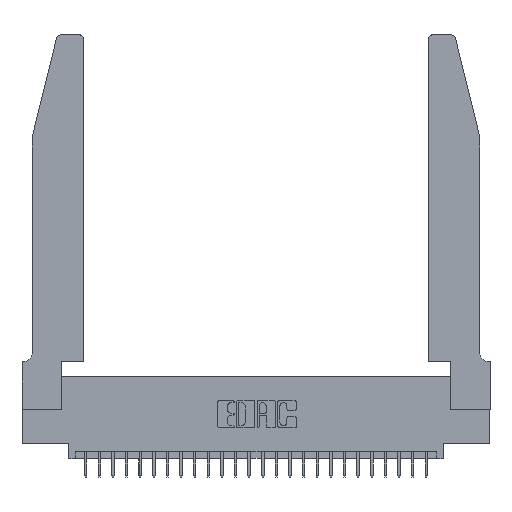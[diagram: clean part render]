
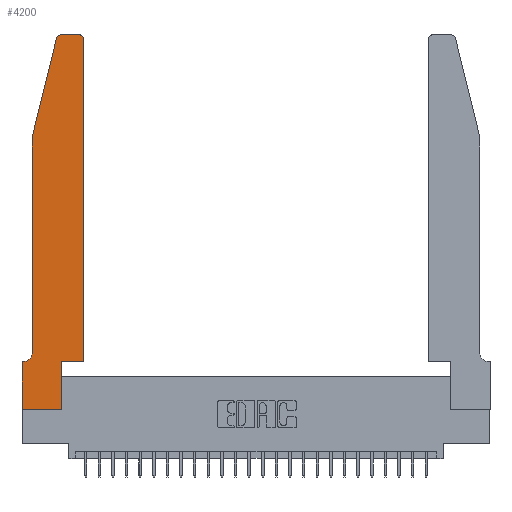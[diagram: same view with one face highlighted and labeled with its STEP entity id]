
A CAD part, top view. The second image highlights one B-rep face of the part: STEP entity #4200.
In plain terms, the highlighted planar face has unit normal (0, 0, 1).
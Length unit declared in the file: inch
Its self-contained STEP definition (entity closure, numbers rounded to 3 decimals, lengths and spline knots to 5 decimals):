
#286 = CARTESIAN_POINT ( 'NONE',  ( 0.4505, 0.35, 0.37 ) ) ;
#693 = ORIENTED_EDGE ( 'NONE', *, *, #15158, .T. ) ;
#902 = EDGE_CURVE ( 'NONE', #25947, #24993, #27378, .T. ) ;
#947 = CARTESIAN_POINT ( 'NONE',  ( 0.0755, 0.42, 0.37 ) ) ;
#1676 = VECTOR ( 'NONE', #17549, 39.37008 ) ;
#1824 = EDGE_CURVE ( 'NONE', #17527, #2844, #10276, .T. ) ;
#1993 = CARTESIAN_POINT ( 'NONE',  ( 0., 0., 0.37 ) ) ;
#2123 = ORIENTED_EDGE ( 'NONE', *, *, #1824, .T. ) ;
#2176 = DIRECTION ( 'NONE',  ( 0., -1., 0. ) ) ;
#2195 = VERTEX_POINT ( 'NONE', #15216 ) ;
#2312 = ORIENTED_EDGE ( 'NONE', *, *, #21171, .T. ) ;
#2531 = LINE ( 'NONE', #286, #27209 ) ;
#2791 = VERTEX_POINT ( 'NONE', #3179 ) ;
#2844 = VERTEX_POINT ( 'NONE', #947 ) ;
#3097 = ORIENTED_EDGE ( 'NONE', *, *, #11349, .T. ) ;
#3179 = CARTESIAN_POINT ( 'NONE',  ( 0., 0.35, 0.37 ) ) ;
#3213 = EDGE_CURVE ( 'NONE', #11040, #15208, #9013, .T. ) ;
#3385 = VECTOR ( 'NONE', #2176, 39.37008 ) ;
#3804 = DIRECTION ( 'NONE',  ( 0., 0., 1. ) ) ;
#3993 = FACE_OUTER_BOUND ( 'NONE', #4051, .T. ) ;
#4051 = EDGE_LOOP ( 'NONE', ( #6333, #10744, #12834, #2123, #693, #6550, #2312, #23709, #12369, #8021, #3097, #27177 ) ) ;
#4200 = ADVANCED_FACE ( 'NONE', ( #3993 ), #25056, .T. ) ;
#5046 = LINE ( 'NONE', #13556, #10520 ) ;
#5375 = VECTOR ( 'NONE', #19959, 39.37008 ) ;
#5408 = CARTESIAN_POINT ( 'NONE',  ( 0., 0., 0.37 ) ) ;
#6083 = CARTESIAN_POINT ( 'NONE',  ( 0.284, 2.75, 0.37 ) ) ;
#6333 = ORIENTED_EDGE ( 'NONE', *, *, #9309, .T. ) ;
#6480 = VERTEX_POINT ( 'NONE', #15811 ) ;
#6550 = ORIENTED_EDGE ( 'NONE', *, *, #9488, .T. ) ;
#6843 = EDGE_CURVE ( 'NONE', #15208, #6895, #2531, .T. ) ;
#6895 = VERTEX_POINT ( 'NONE', #17301 ) ;
#7716 = DIRECTION ( 'NONE',  ( 1., 0., 0. ) ) ;
#8021 = ORIENTED_EDGE ( 'NONE', *, *, #6843, .T. ) ;
#8030 = EDGE_CURVE ( 'NONE', #6480, #11040, #12855, .T. ) ;
#8060 = VECTOR ( 'NONE', #18985, 39.37008 ) ;
#8139 = EDGE_CURVE ( 'NONE', #24993, #17527, #13684, .T. ) ;
#9013 = LINE ( 'NONE', #17930, #10555 ) ;
#9209 = DIRECTION ( 'NONE',  ( -1., 0., 0. ) ) ;
#9309 = EDGE_CURVE ( 'NONE', #2195, #25947, #13139, .T. ) ;
#9488 = EDGE_CURVE ( 'NONE', #26459, #2791, #5046, .T. ) ;
#10028 = CARTESIAN_POINT ( 'NONE',  ( 0.2865, 0.35, 0.37 ) ) ;
#10276 = LINE ( 'NONE', #10548, #3385 ) ;
#10520 = VECTOR ( 'NONE', #25966, 39.37008 ) ;
#10548 = CARTESIAN_POINT ( 'NONE',  ( 0.0755, 2., 0.37 ) ) ;
#10555 = VECTOR ( 'NONE', #21689, 39.37008 ) ;
#10564 = DIRECTION ( 'NONE',  ( 0., 0., 1. ) ) ;
#10744 = ORIENTED_EDGE ( 'NONE', *, *, #902, .T. ) ;
#11040 = VERTEX_POINT ( 'NONE', #14069 ) ;
#11300 = CARTESIAN_POINT ( 'NONE',  ( 0.0055, 0.42, 0.37 ) ) ;
#11349 = EDGE_CURVE ( 'NONE', #6895, #15377, #17132, .T. ) ;
#11638 = CIRCLE ( 'NONE', #13412, 0.07 ) ;
#12369 = ORIENTED_EDGE ( 'NONE', *, *, #3213, .T. ) ;
#12834 = ORIENTED_EDGE ( 'NONE', *, *, #8139, .T. ) ;
#12855 = LINE ( 'NONE', #1993, #8060 ) ;
#13139 = LINE ( 'NONE', #15234, #19622 ) ;
#13275 = CARTESIAN_POINT ( 'NONE',  ( 0.0755, 2., 0.37 ) ) ;
#13412 = AXIS2_PLACEMENT_3D ( 'NONE', #11300, #19797, #9209 ) ;
#13556 = CARTESIAN_POINT ( 'NONE',  ( 0.0755, 0.35, 0.37 ) ) ;
#13684 = LINE ( 'NONE', #13275, #5375 ) ;
#13692 = AXIS2_PLACEMENT_3D ( 'NONE', #20457, #16407, #14045 ) ;
#14045 = DIRECTION ( 'NONE',  ( 1., 0., 0. ) ) ;
#14069 = CARTESIAN_POINT ( 'NONE',  ( 0.2865, 0., 0.37 ) ) ;
#15106 = CARTESIAN_POINT ( 'NONE',  ( 0.0755, 2., 0.37 ) ) ;
#15158 = EDGE_CURVE ( 'NONE', #2844, #26459, #11638, .T. ) ;
#15208 = VERTEX_POINT ( 'NONE', #10028 ) ;
#15216 = CARTESIAN_POINT ( 'NONE',  ( 0.4205, 2.75, 0.37 ) ) ;
#15234 = CARTESIAN_POINT ( 'NONE',  ( 0.2605, 2.75, 0.37 ) ) ;
#15377 = VERTEX_POINT ( 'NONE', #15447 ) ;
#15447 = CARTESIAN_POINT ( 'NONE',  ( 0.4505, 2.72, 0.37 ) ) ;
#15811 = CARTESIAN_POINT ( 'NONE',  ( 0., 0., 0.37 ) ) ;
#16407 = DIRECTION ( 'NONE',  ( 0., 0., 1. ) ) ;
#17132 = LINE ( 'NONE', #25905, #1676 ) ;
#17301 = CARTESIAN_POINT ( 'NONE',  ( 0.4505, 0.35, 0.37 ) ) ;
#17527 = VERTEX_POINT ( 'NONE', #15106 ) ;
#17549 = DIRECTION ( 'NONE',  ( 0., 1., 0. ) ) ;
#17585 = AXIS2_PLACEMENT_3D ( 'NONE', #22511, #3804, #7716 ) ;
#17930 = CARTESIAN_POINT ( 'NONE',  ( 0.2865, 0.35, 0.37 ) ) ;
#18617 = CIRCLE ( 'NONE', #21754, 0.03 ) ;
#18917 = DIRECTION ( 'NONE',  ( 1., 0., 0. ) ) ;
#18985 = DIRECTION ( 'NONE',  ( 1., 0., 0. ) ) ;
#19344 = VECTOR ( 'NONE', #24652, 39.37008 ) ;
#19622 = VECTOR ( 'NONE', #27492, 39.37008 ) ;
#19683 = DIRECTION ( 'NONE',  ( 1., 0., 0. ) ) ;
#19797 = DIRECTION ( 'NONE',  ( 0., 0., -1. ) ) ;
#19959 = DIRECTION ( 'NONE',  ( -0.239, -0.971, 0. ) ) ;
#20061 = CARTESIAN_POINT ( 'NONE',  ( 0.25487, 2.72718, 0.37 ) ) ;
#20457 = CARTESIAN_POINT ( 'NONE',  ( 0., 0.35, 0.37 ) ) ;
#21171 = EDGE_CURVE ( 'NONE', #2791, #6480, #24522, .T. ) ;
#21689 = DIRECTION ( 'NONE',  ( 0., 1., 0. ) ) ;
#21754 = AXIS2_PLACEMENT_3D ( 'NONE', #25334, #10564, #18917 ) ;
#22511 = CARTESIAN_POINT ( 'NONE',  ( 0.284, 2.72, 0.37 ) ) ;
#23709 = ORIENTED_EDGE ( 'NONE', *, *, #8030, .T. ) ;
#24522 = LINE ( 'NONE', #5408, #19344 ) ;
#24652 = DIRECTION ( 'NONE',  ( 0., -1., 0. ) ) ;
#24993 = VERTEX_POINT ( 'NONE', #20061 ) ;
#25056 = PLANE ( 'NONE',  #13692 ) ;
#25173 = EDGE_CURVE ( 'NONE', #15377, #2195, #18617, .T. ) ;
#25334 = CARTESIAN_POINT ( 'NONE',  ( 0.4205, 2.72, 0.37 ) ) ;
#25905 = CARTESIAN_POINT ( 'NONE',  ( 0.4505, 0.35, 0.37 ) ) ;
#25947 = VERTEX_POINT ( 'NONE', #6083 ) ;
#25966 = DIRECTION ( 'NONE',  ( -1., 0., 0. ) ) ;
#26459 = VERTEX_POINT ( 'NONE', #27252 ) ;
#27177 = ORIENTED_EDGE ( 'NONE', *, *, #25173, .T. ) ;
#27209 = VECTOR ( 'NONE', #19683, 39.37008 ) ;
#27252 = CARTESIAN_POINT ( 'NONE',  ( 0.0055, 0.35, 0.37 ) ) ;
#27378 = CIRCLE ( 'NONE', #17585, 0.03 ) ;
#27492 = DIRECTION ( 'NONE',  ( -1., 0., 0. ) ) ;
